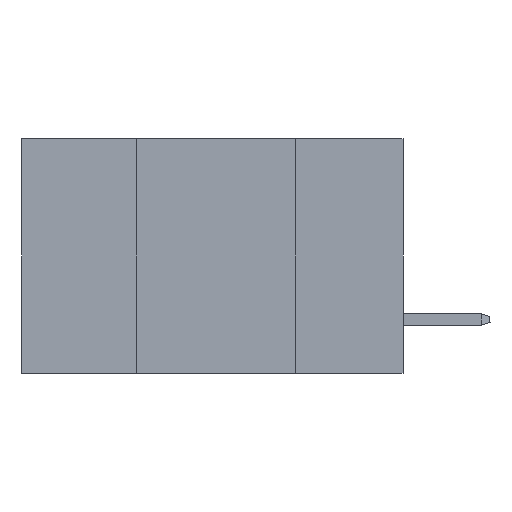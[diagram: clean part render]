
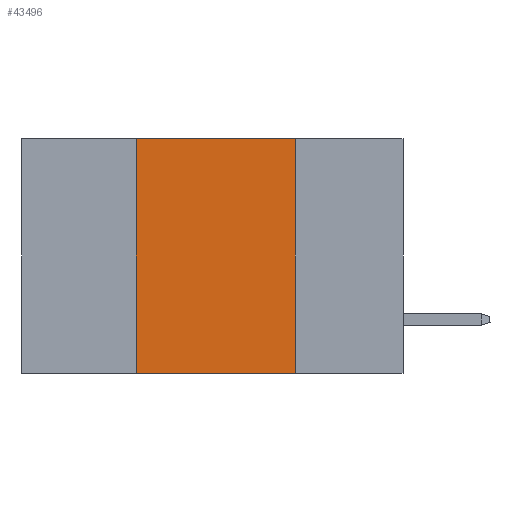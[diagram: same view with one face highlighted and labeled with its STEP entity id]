
A CAD part, left-side view. The second image highlights one B-rep face of the part: STEP entity #43496.
In plain terms, the highlighted planar face has unit normal (-1, 0, 0).
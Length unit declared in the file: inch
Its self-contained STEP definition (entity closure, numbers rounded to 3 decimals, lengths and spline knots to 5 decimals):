
#267 = CARTESIAN_POINT ( 'NONE',  ( 0., 0.42, 0. ) ) ;
#1777 = EDGE_CURVE ( 'NONE', #22111, #14341, #33413, .T. ) ;
#5342 = ORIENTED_EDGE ( 'NONE', *, *, #1777, .F. ) ;
#6305 = VERTEX_POINT ( 'NONE', #22456 ) ;
#7730 = CARTESIAN_POINT ( 'NONE',  ( 0., 0.17, 0. ) ) ;
#8999 = ORIENTED_EDGE ( 'NONE', *, *, #32752, .T. ) ;
#11142 = CARTESIAN_POINT ( 'NONE',  ( 0., 0.42, 0. ) ) ;
#11335 = LINE ( 'NONE', #11809, #47013 ) ;
#11809 = CARTESIAN_POINT ( 'NONE',  ( 0., 0.6, 0. ) ) ;
#12200 = EDGE_LOOP ( 'NONE', ( #31757, #39344, #5342, #8999 ) ) ;
#13556 = CARTESIAN_POINT ( 'NONE',  ( 0., 0.17, 0. ) ) ;
#14341 = VERTEX_POINT ( 'NONE', #267 ) ;
#14552 = AXIS2_PLACEMENT_3D ( 'NONE', #43495, #32365, #46884 ) ;
#17309 = EDGE_CURVE ( 'NONE', #46071, #6305, #40886, .T. ) ;
#17374 = FACE_OUTER_BOUND ( 'NONE', #12200, .T. ) ;
#18857 = DIRECTION ( 'NONE',  ( 0., -1., 0. ) ) ;
#21969 = PLANE ( 'NONE',  #14552 ) ;
#22039 = DIRECTION ( 'NONE',  ( 0., 0., -1. ) ) ;
#22111 = VERTEX_POINT ( 'NONE', #29588 ) ;
#22456 = CARTESIAN_POINT ( 'NONE',  ( 0., 0.17, -0.37 ) ) ;
#23821 = CARTESIAN_POINT ( 'NONE',  ( 0., 0.6, -0.37 ) ) ;
#29588 = CARTESIAN_POINT ( 'NONE',  ( 0., 0.42, -0.37 ) ) ;
#30813 = VECTOR ( 'NONE', #34490, 39.37008 ) ;
#31324 = LINE ( 'NONE', #23821, #30813 ) ;
#31757 = ORIENTED_EDGE ( 'NONE', *, *, #17309, .F. ) ;
#32237 = EDGE_CURVE ( 'NONE', #14341, #46071, #11335, .T. ) ;
#32365 = DIRECTION ( 'NONE',  ( 1., 0., 0. ) ) ;
#32752 = EDGE_CURVE ( 'NONE', #22111, #6305, #31324, .T. ) ;
#33413 = LINE ( 'NONE', #11142, #42454 ) ;
#34490 = DIRECTION ( 'NONE',  ( 0., -1., 0. ) ) ;
#38561 = VECTOR ( 'NONE', #22039, 39.37008 ) ;
#39344 = ORIENTED_EDGE ( 'NONE', *, *, #32237, .F. ) ;
#40661 = DIRECTION ( 'NONE',  ( 0., 0., 1. ) ) ;
#40886 = LINE ( 'NONE', #7730, #38561 ) ;
#42454 = VECTOR ( 'NONE', #40661, 39.37008 ) ;
#43495 = CARTESIAN_POINT ( 'NONE',  ( 0., 0.6, 0. ) ) ;
#43496 = ADVANCED_FACE ( 'NONE', ( #17374 ), #21969, .F. ) ;
#46071 = VERTEX_POINT ( 'NONE', #13556 ) ;
#46884 = DIRECTION ( 'NONE',  ( 0., 0., -1. ) ) ;
#47013 = VECTOR ( 'NONE', #18857, 39.37008 ) ;
